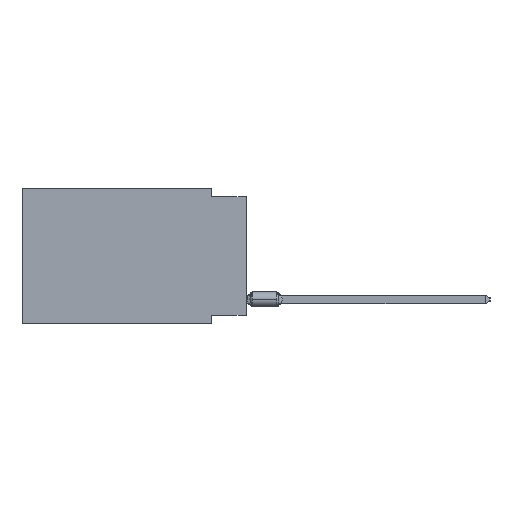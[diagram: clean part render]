
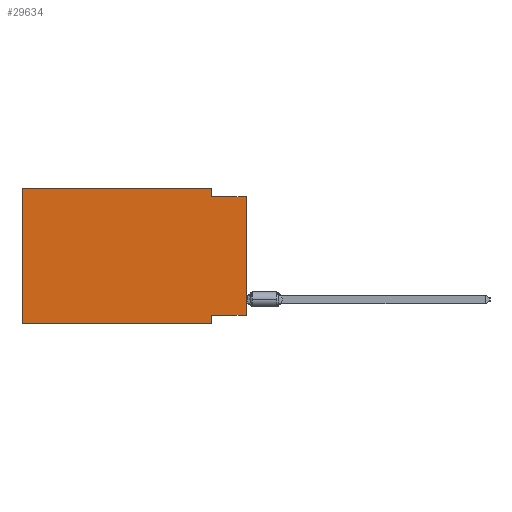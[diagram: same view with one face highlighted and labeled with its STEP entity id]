
A CAD part, left-side view. The second image highlights one B-rep face of the part: STEP entity #29634.
In plain terms, the highlighted planar face has unit normal (-1, 0, 0).
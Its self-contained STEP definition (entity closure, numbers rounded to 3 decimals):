
#161 = CARTESIAN_POINT ( 'NONE',  ( 0., 2.54, -9.906 ) ) ;
#1252 = PLANE ( 'NONE',  #25559 ) ;
#1449 = DIRECTION ( 'NONE',  ( 0., 0., 1. ) ) ;
#2377 = VERTEX_POINT ( 'NONE', #28942 ) ;
#3030 = CARTESIAN_POINT ( 'NONE',  ( 0., 16.383, 0. ) ) ;
#3183 = LINE ( 'NONE', #28746, #7113 ) ;
#3283 = DIRECTION ( 'NONE',  ( 0., 0., -1. ) ) ;
#4858 = VECTOR ( 'NONE', #3283, 1000. ) ;
#5319 = DIRECTION ( 'NONE',  ( 0., 1., 0. ) ) ;
#5748 = VERTEX_POINT ( 'NONE', #21522 ) ;
#5803 = ORIENTED_EDGE ( 'NONE', *, *, #6200, .F. ) ;
#5943 = VECTOR ( 'NONE', #34749, 1000. ) ;
#6200 = EDGE_CURVE ( 'NONE', #2377, #5748, #8682, .T. ) ;
#6571 = LINE ( 'NONE', #20816, #31145 ) ;
#7045 = CARTESIAN_POINT ( 'NONE',  ( 0., 2.54, -9.271 ) ) ;
#7113 = VECTOR ( 'NONE', #31100, 1000. ) ;
#7165 = EDGE_CURVE ( 'NONE', #23653, #11931, #11322, .T. ) ;
#7559 = ORIENTED_EDGE ( 'NONE', *, *, #20065, .F. ) ;
#8536 = EDGE_CURVE ( 'NONE', #17410, #23653, #30158, .T. ) ;
#8682 = LINE ( 'NONE', #3030, #28132 ) ;
#9477 = DIRECTION ( 'NONE',  ( 0., 0., -1. ) ) ;
#9660 = DIRECTION ( 'NONE',  ( 1., 0., 0. ) ) ;
#10839 = DIRECTION ( 'NONE',  ( 0., -1., 0. ) ) ;
#10866 = CARTESIAN_POINT ( 'NONE',  ( 0., 2.54, 0. ) ) ;
#11167 = ORIENTED_EDGE ( 'NONE', *, *, #18551, .T. ) ;
#11208 = EDGE_LOOP ( 'NONE', ( #28226, #15125, #7559, #23973, #5803, #11167, #21625, #33753 ) ) ;
#11322 = LINE ( 'NONE', #25946, #4858 ) ;
#11931 = VERTEX_POINT ( 'NONE', #161 ) ;
#12329 = LINE ( 'NONE', #12513, #5943 ) ;
#12513 = CARTESIAN_POINT ( 'NONE',  ( 0., 2.54, 0. ) ) ;
#13140 = VECTOR ( 'NONE', #10839, 1000. ) ;
#13992 = DIRECTION ( 'NONE',  ( 0., 0., 1. ) ) ;
#15125 = ORIENTED_EDGE ( 'NONE', *, *, #33106, .F. ) ;
#17410 = VERTEX_POINT ( 'NONE', #33237 ) ;
#18056 = CARTESIAN_POINT ( 'NONE',  ( 0., 16.383, 0. ) ) ;
#18423 = CARTESIAN_POINT ( 'NONE',  ( 0., 2.54, -0.635 ) ) ;
#18551 = EDGE_CURVE ( 'NONE', #2377, #11931, #21561, .T. ) ;
#18957 = VECTOR ( 'NONE', #5319, 1000. ) ;
#19069 = LINE ( 'NONE', #28182, #13140 ) ;
#19409 = CARTESIAN_POINT ( 'NONE',  ( 0., 0., -9.271 ) ) ;
#20065 = EDGE_CURVE ( 'NONE', #29121, #29779, #12329, .T. ) ;
#20816 = CARTESIAN_POINT ( 'NONE',  ( 0., 0., 0. ) ) ;
#21467 = CARTESIAN_POINT ( 'NONE',  ( 0., 0., -0.635 ) ) ;
#21522 = CARTESIAN_POINT ( 'NONE',  ( 0., 16.383, 0. ) ) ;
#21561 = LINE ( 'NONE', #32312, #23419 ) ;
#21625 = ORIENTED_EDGE ( 'NONE', *, *, #7165, .F. ) ;
#22449 = EDGE_CURVE ( 'NONE', #17410, #23637, #6571, .T. ) ;
#23419 = VECTOR ( 'NONE', #32667, 1000. ) ;
#23533 = EDGE_CURVE ( 'NONE', #5748, #29121, #19069, .T. ) ;
#23637 = VERTEX_POINT ( 'NONE', #21467 ) ;
#23653 = VERTEX_POINT ( 'NONE', #7045 ) ;
#23973 = ORIENTED_EDGE ( 'NONE', *, *, #23533, .F. ) ;
#25559 = AXIS2_PLACEMENT_3D ( 'NONE', #18056, #9660, #9477 ) ;
#25946 = CARTESIAN_POINT ( 'NONE',  ( 0., 2.54, -9.906 ) ) ;
#28132 = VECTOR ( 'NONE', #13992, 1000. ) ;
#28182 = CARTESIAN_POINT ( 'NONE',  ( 0., 16.383, 0. ) ) ;
#28226 = ORIENTED_EDGE ( 'NONE', *, *, #22449, .T. ) ;
#28746 = CARTESIAN_POINT ( 'NONE',  ( 0., 0., -0.635 ) ) ;
#28942 = CARTESIAN_POINT ( 'NONE',  ( 0., 16.383, -9.906 ) ) ;
#29121 = VERTEX_POINT ( 'NONE', #10866 ) ;
#29634 = ADVANCED_FACE ( 'NONE', ( #34292 ), #1252, .F. ) ;
#29779 = VERTEX_POINT ( 'NONE', #18423 ) ;
#30158 = LINE ( 'NONE', #19409, #18957 ) ;
#31100 = DIRECTION ( 'NONE',  ( 0., -1., 0. ) ) ;
#31145 = VECTOR ( 'NONE', #1449, 1000. ) ;
#32312 = CARTESIAN_POINT ( 'NONE',  ( 0., 16.383, -9.906 ) ) ;
#32667 = DIRECTION ( 'NONE',  ( 0., -1., 0. ) ) ;
#33106 = EDGE_CURVE ( 'NONE', #29779, #23637, #3183, .T. ) ;
#33237 = CARTESIAN_POINT ( 'NONE',  ( 0., 0., -9.271 ) ) ;
#33753 = ORIENTED_EDGE ( 'NONE', *, *, #8536, .F. ) ;
#34292 = FACE_OUTER_BOUND ( 'NONE', #11208, .T. ) ;
#34749 = DIRECTION ( 'NONE',  ( 0., 0., -1. ) ) ;
